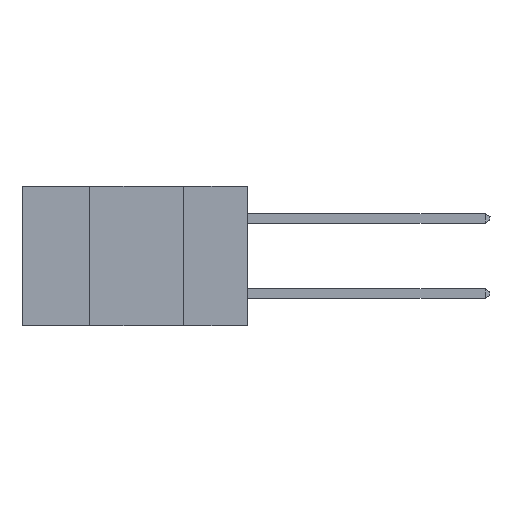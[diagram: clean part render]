
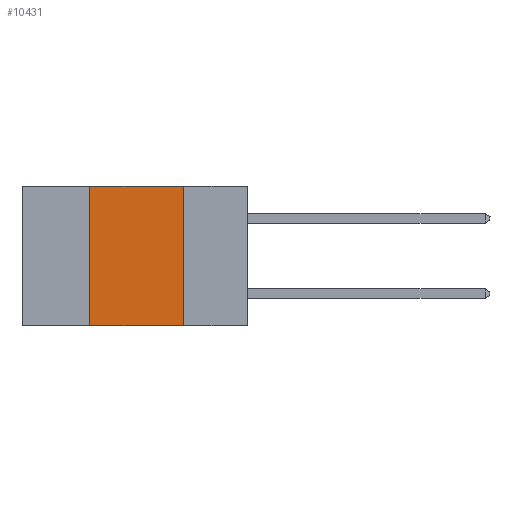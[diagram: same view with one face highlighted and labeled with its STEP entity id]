
A CAD part, left-side view. The second image highlights one B-rep face of the part: STEP entity #10431.
In plain terms, the highlighted planar face has unit normal (-1, 0, 0).
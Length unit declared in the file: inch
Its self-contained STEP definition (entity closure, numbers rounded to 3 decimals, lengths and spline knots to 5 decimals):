
#427 = VECTOR ( 'NONE', #2212, 39.37008 ) ;
#592 = CARTESIAN_POINT ( 'NONE',  ( 0., 0.42, 0. ) ) ;
#603 = CARTESIAN_POINT ( 'NONE',  ( 0., 0.17, 0. ) ) ;
#1342 = CARTESIAN_POINT ( 'NONE',  ( 0., 0.42, 0. ) ) ;
#1767 = EDGE_CURVE ( 'NONE', #15767, #16409, #4986, .T. ) ;
#1778 = LINE ( 'NONE', #5807, #10741 ) ;
#2212 = DIRECTION ( 'NONE',  ( 0., 0., -1. ) ) ;
#4016 = VECTOR ( 'NONE', #4613, 39.37008 ) ;
#4041 = AXIS2_PLACEMENT_3D ( 'NONE', #13597, #13430, #7134 ) ;
#4463 = ORIENTED_EDGE ( 'NONE', *, *, #10436, .F. ) ;
#4613 = DIRECTION ( 'NONE',  ( 0., -1., 0. ) ) ;
#4726 = LINE ( 'NONE', #592, #10352 ) ;
#4986 = LINE ( 'NONE', #5872, #427 ) ;
#5807 = CARTESIAN_POINT ( 'NONE',  ( 0., 0.6, 0. ) ) ;
#5872 = CARTESIAN_POINT ( 'NONE',  ( 0., 0.17, 0. ) ) ;
#5989 = ORIENTED_EDGE ( 'NONE', *, *, #1767, .F. ) ;
#6243 = VERTEX_POINT ( 'NONE', #1342 ) ;
#6727 = FACE_OUTER_BOUND ( 'NONE', #10666, .T. ) ;
#7134 = DIRECTION ( 'NONE',  ( 0., 0., -1. ) ) ;
#8722 = EDGE_CURVE ( 'NONE', #15860, #16409, #13408, .T. ) ;
#9389 = ORIENTED_EDGE ( 'NONE', *, *, #8722, .T. ) ;
#9609 = CARTESIAN_POINT ( 'NONE',  ( 0., 0.6, -0.37 ) ) ;
#10319 = CARTESIAN_POINT ( 'NONE',  ( 0., 0.42, -0.37 ) ) ;
#10352 = VECTOR ( 'NONE', #13545, 39.37008 ) ;
#10392 = EDGE_CURVE ( 'NONE', #6243, #15767, #1778, .T. ) ;
#10431 = ADVANCED_FACE ( 'NONE', ( #6727 ), #15938, .F. ) ;
#10436 = EDGE_CURVE ( 'NONE', #15860, #6243, #4726, .T. ) ;
#10666 = EDGE_LOOP ( 'NONE', ( #5989, #12040, #4463, #9389 ) ) ;
#10741 = VECTOR ( 'NONE', #14795, 39.37008 ) ;
#11479 = CARTESIAN_POINT ( 'NONE',  ( 0., 0.17, -0.37 ) ) ;
#12040 = ORIENTED_EDGE ( 'NONE', *, *, #10392, .F. ) ;
#13408 = LINE ( 'NONE', #9609, #4016 ) ;
#13430 = DIRECTION ( 'NONE',  ( 1., 0., 0. ) ) ;
#13545 = DIRECTION ( 'NONE',  ( 0., 0., 1. ) ) ;
#13597 = CARTESIAN_POINT ( 'NONE',  ( 0., 0.6, 0. ) ) ;
#14795 = DIRECTION ( 'NONE',  ( 0., -1., 0. ) ) ;
#15767 = VERTEX_POINT ( 'NONE', #603 ) ;
#15860 = VERTEX_POINT ( 'NONE', #10319 ) ;
#15938 = PLANE ( 'NONE',  #4041 ) ;
#16409 = VERTEX_POINT ( 'NONE', #11479 ) ;
